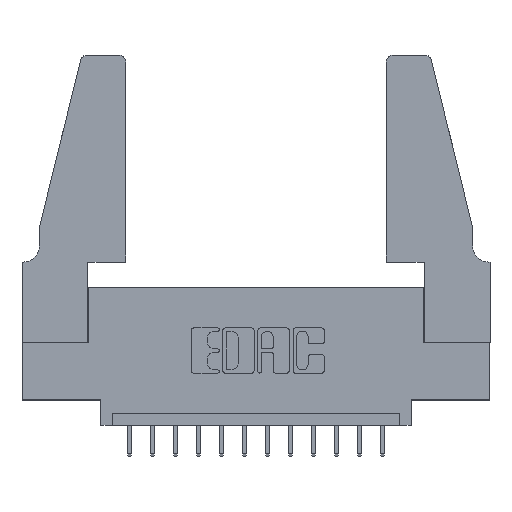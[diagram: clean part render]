
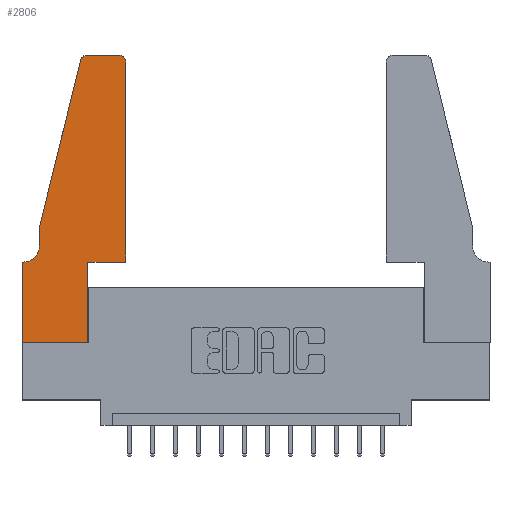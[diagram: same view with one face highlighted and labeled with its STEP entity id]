
A CAD part, top view. The second image highlights one B-rep face of the part: STEP entity #2806.
In plain terms, the highlighted planar face has unit normal (0, 0, 1).
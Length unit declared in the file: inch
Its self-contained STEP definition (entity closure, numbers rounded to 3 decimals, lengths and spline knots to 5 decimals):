
#221 = EDGE_CURVE ( 'NONE', #14577, #12482, #8613, .T. ) ;
#504 = LINE ( 'NONE', #12587, #5039 ) ;
#581 = AXIS2_PLACEMENT_3D ( 'NONE', #592, #2943, #13565 ) ;
#585 = VECTOR ( 'NONE', #9942, 39.37008 ) ;
#592 = CARTESIAN_POINT ( 'NONE',  ( 0.284, 1.22, 0.37 ) ) ;
#662 = DIRECTION ( 'NONE',  ( -0.239, -0.971, 0. ) ) ;
#698 = PLANE ( 'NONE',  #12312 ) ;
#833 = CIRCLE ( 'NONE', #581, 0.03 ) ;
#935 = ORIENTED_EDGE ( 'NONE', *, *, #4483, .T. ) ;
#990 = DIRECTION ( 'NONE',  ( 0., 1., 0. ) ) ;
#1727 = VERTEX_POINT ( 'NONE', #10336 ) ;
#1765 = CARTESIAN_POINT ( 'NONE',  ( 0., 0., 0.37 ) ) ;
#1774 = EDGE_LOOP ( 'NONE', ( #5037, #935, #9348, #9753, #11688, #13032, #2518, #14216, #7914, #13111, #11417, #2029 ) ) ;
#2006 = EDGE_CURVE ( 'NONE', #13839, #1727, #5569, .T. ) ;
#2012 = DIRECTION ( 'NONE',  ( 0., 0., 1. ) ) ;
#2029 = ORIENTED_EDGE ( 'NONE', *, *, #2006, .T. ) ;
#2386 = VECTOR ( 'NONE', #7444, 39.37008 ) ;
#2443 = VERTEX_POINT ( 'NONE', #12434 ) ;
#2518 = ORIENTED_EDGE ( 'NONE', *, *, #3287, .T. ) ;
#2550 = CARTESIAN_POINT ( 'NONE',  ( 0.0755, 0.5, 0.37 ) ) ;
#2686 = EDGE_CURVE ( 'NONE', #14979, #12662, #3986, .T. ) ;
#2806 = ADVANCED_FACE ( 'NONE', ( #3199 ), #698, .T. ) ;
#2943 = DIRECTION ( 'NONE',  ( 0., 0., 1. ) ) ;
#2950 = CARTESIAN_POINT ( 'NONE',  ( 0.2605, 1.25, 0.37 ) ) ;
#3199 = FACE_OUTER_BOUND ( 'NONE', #1774, .T. ) ;
#3287 = EDGE_CURVE ( 'NONE', #12662, #13285, #11345, .T. ) ;
#3582 = EDGE_CURVE ( 'NONE', #7821, #3742, #3801, .T. ) ;
#3742 = VERTEX_POINT ( 'NONE', #12739 ) ;
#3801 = LINE ( 'NONE', #8681, #2386 ) ;
#3842 = VECTOR ( 'NONE', #990, 39.37008 ) ;
#3986 = LINE ( 'NONE', #7713, #8164 ) ;
#4282 = CARTESIAN_POINT ( 'NONE',  ( 0.0755, 0.5, 0.37 ) ) ;
#4295 = CARTESIAN_POINT ( 'NONE',  ( 0.4505, 0.35, 0.37 ) ) ;
#4319 = CARTESIAN_POINT ( 'NONE',  ( 0.0755, 0.42, 0.37 ) ) ;
#4483 = EDGE_CURVE ( 'NONE', #6870, #12841, #833, .T. ) ;
#4686 = EDGE_CURVE ( 'NONE', #2443, #13839, #9239, .T. ) ;
#4869 = VECTOR ( 'NONE', #13959, 39.37008 ) ;
#5037 = ORIENTED_EDGE ( 'NONE', *, *, #7131, .T. ) ;
#5039 = VECTOR ( 'NONE', #662, 39.37008 ) ;
#5166 = CARTESIAN_POINT ( 'NONE',  ( 0.4205, 1.22, 0.37 ) ) ;
#5366 = CIRCLE ( 'NONE', #11842, 0.07 ) ;
#5538 = VECTOR ( 'NONE', #9043, 39.37008 ) ;
#5569 = CIRCLE ( 'NONE', #7576, 0.03 ) ;
#5618 = LINE ( 'NONE', #4295, #5538 ) ;
#5638 = CARTESIAN_POINT ( 'NONE',  ( 0., 0.35, 0.37 ) ) ;
#5760 = DIRECTION ( 'NONE',  ( 1., 0., 0. ) ) ;
#6228 = EDGE_CURVE ( 'NONE', #12841, #14577, #504, .T. ) ;
#6562 = DIRECTION ( 'NONE',  ( 1., 0., 0. ) ) ;
#6604 = CARTESIAN_POINT ( 'NONE',  ( 0.0055, 0.35, 0.37 ) ) ;
#6870 = VERTEX_POINT ( 'NONE', #10959 ) ;
#7131 = EDGE_CURVE ( 'NONE', #1727, #6870, #12607, .T. ) ;
#7272 = CARTESIAN_POINT ( 'NONE',  ( 0.2865, 0., 0.37 ) ) ;
#7444 = DIRECTION ( 'NONE',  ( 0., 1., 0. ) ) ;
#7576 = AXIS2_PLACEMENT_3D ( 'NONE', #5166, #12495, #6562 ) ;
#7713 = CARTESIAN_POINT ( 'NONE',  ( 0.0755, 0.35, 0.37 ) ) ;
#7821 = VERTEX_POINT ( 'NONE', #7272 ) ;
#7914 = ORIENTED_EDGE ( 'NONE', *, *, #3582, .T. ) ;
#7938 = DIRECTION ( 'NONE',  ( 1., 0., 0. ) ) ;
#7949 = LINE ( 'NONE', #12711, #14190 ) ;
#7990 = EDGE_CURVE ( 'NONE', #3742, #2443, #5618, .T. ) ;
#8161 = CARTESIAN_POINT ( 'NONE',  ( 0.4505, 1.22, 0.37 ) ) ;
#8164 = VECTOR ( 'NONE', #11051, 39.37008 ) ;
#8613 = LINE ( 'NONE', #2550, #14566 ) ;
#8681 = CARTESIAN_POINT ( 'NONE',  ( 0.2865, 0.35, 0.37 ) ) ;
#9043 = DIRECTION ( 'NONE',  ( 1., 0., 0. ) ) ;
#9239 = LINE ( 'NONE', #11662, #3842 ) ;
#9348 = ORIENTED_EDGE ( 'NONE', *, *, #6228, .T. ) ;
#9441 = DIRECTION ( 'NONE',  ( 0., 0., -1. ) ) ;
#9556 = DIRECTION ( 'NONE',  ( 0., -1., 0. ) ) ;
#9753 = ORIENTED_EDGE ( 'NONE', *, *, #221, .T. ) ;
#9762 = CARTESIAN_POINT ( 'NONE',  ( 0.25487, 1.22718, 0.37 ) ) ;
#9942 = DIRECTION ( 'NONE',  ( -1., 0., 0. ) ) ;
#10263 = CARTESIAN_POINT ( 'NONE',  ( 0., 0.35, 0.37 ) ) ;
#10336 = CARTESIAN_POINT ( 'NONE',  ( 0.4205, 1.25, 0.37 ) ) ;
#10959 = CARTESIAN_POINT ( 'NONE',  ( 0.284, 1.25, 0.37 ) ) ;
#11014 = EDGE_CURVE ( 'NONE', #12482, #14979, #5366, .T. ) ;
#11051 = DIRECTION ( 'NONE',  ( -1., 0., 0. ) ) ;
#11345 = LINE ( 'NONE', #1765, #4869 ) ;
#11417 = ORIENTED_EDGE ( 'NONE', *, *, #4686, .T. ) ;
#11662 = CARTESIAN_POINT ( 'NONE',  ( 0.4505, 0.35, 0.37 ) ) ;
#11688 = ORIENTED_EDGE ( 'NONE', *, *, #11014, .T. ) ;
#11842 = AXIS2_PLACEMENT_3D ( 'NONE', #14162, #9441, #11861 ) ;
#11861 = DIRECTION ( 'NONE',  ( -1., 0., 0. ) ) ;
#12312 = AXIS2_PLACEMENT_3D ( 'NONE', #10263, #2012, #7938 ) ;
#12434 = CARTESIAN_POINT ( 'NONE',  ( 0.4505, 0.35, 0.37 ) ) ;
#12482 = VERTEX_POINT ( 'NONE', #4319 ) ;
#12495 = DIRECTION ( 'NONE',  ( 0., 0., 1. ) ) ;
#12587 = CARTESIAN_POINT ( 'NONE',  ( 0.0755, 0.5, 0.37 ) ) ;
#12607 = LINE ( 'NONE', #2950, #585 ) ;
#12662 = VERTEX_POINT ( 'NONE', #5638 ) ;
#12711 = CARTESIAN_POINT ( 'NONE',  ( 0., 0., 0.37 ) ) ;
#12739 = CARTESIAN_POINT ( 'NONE',  ( 0.2865, 0.35, 0.37 ) ) ;
#12841 = VERTEX_POINT ( 'NONE', #9762 ) ;
#13032 = ORIENTED_EDGE ( 'NONE', *, *, #2686, .T. ) ;
#13111 = ORIENTED_EDGE ( 'NONE', *, *, #7990, .T. ) ;
#13285 = VERTEX_POINT ( 'NONE', #13517 ) ;
#13517 = CARTESIAN_POINT ( 'NONE',  ( 0., 0., 0.37 ) ) ;
#13565 = DIRECTION ( 'NONE',  ( 1., 0., 0. ) ) ;
#13839 = VERTEX_POINT ( 'NONE', #8161 ) ;
#13959 = DIRECTION ( 'NONE',  ( 0., -1., 0. ) ) ;
#14162 = CARTESIAN_POINT ( 'NONE',  ( 0.0055, 0.42, 0.37 ) ) ;
#14190 = VECTOR ( 'NONE', #5760, 39.37008 ) ;
#14216 = ORIENTED_EDGE ( 'NONE', *, *, #14770, .T. ) ;
#14566 = VECTOR ( 'NONE', #9556, 39.37008 ) ;
#14577 = VERTEX_POINT ( 'NONE', #4282 ) ;
#14770 = EDGE_CURVE ( 'NONE', #13285, #7821, #7949, .T. ) ;
#14979 = VERTEX_POINT ( 'NONE', #6604 ) ;
